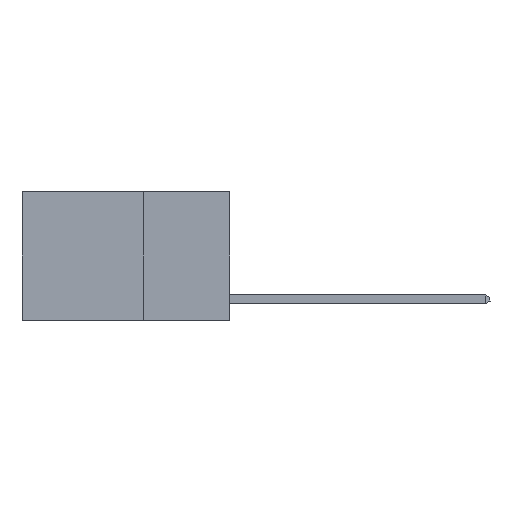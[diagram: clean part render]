
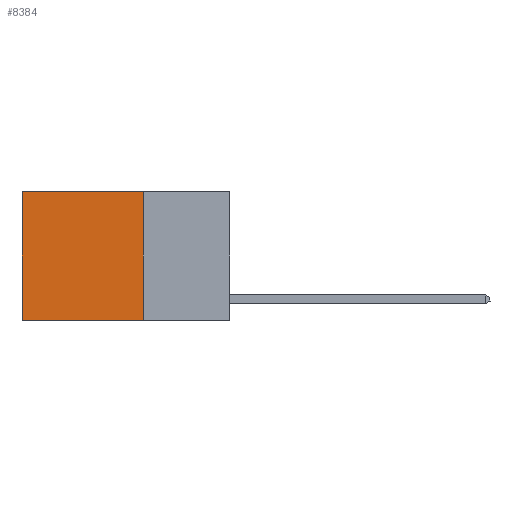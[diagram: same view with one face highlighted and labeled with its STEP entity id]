
A CAD part, left-side view. The second image highlights one B-rep face of the part: STEP entity #8384.
In plain terms, the highlighted planar face has unit normal (-1, 0, 0).
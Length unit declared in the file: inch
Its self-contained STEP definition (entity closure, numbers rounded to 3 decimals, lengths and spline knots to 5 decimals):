
#756 = DIRECTION ( 'NONE',  ( 1., 0., 0. ) ) ;
#1683 = ORIENTED_EDGE ( 'NONE', *, *, #12003, .F. ) ;
#1758 = VECTOR ( 'NONE', #3280, 39.37008 ) ;
#2076 = VECTOR ( 'NONE', #7123, 39.37008 ) ;
#2706 = AXIS2_PLACEMENT_3D ( 'NONE', #3637, #756, #6891 ) ;
#3280 = DIRECTION ( 'NONE',  ( 0., 1., 0. ) ) ;
#3371 = VERTEX_POINT ( 'NONE', #11591 ) ;
#3637 = CARTESIAN_POINT ( 'NONE',  ( 0.2625, 0.25, 0. ) ) ;
#4453 = CARTESIAN_POINT ( 'NONE',  ( 0.2625, 0.6, 0. ) ) ;
#4506 = EDGE_CURVE ( 'NONE', #8704, #18616, #5095, .T. ) ;
#5095 = LINE ( 'NONE', #8259, #14985 ) ;
#5238 = ORIENTED_EDGE ( 'NONE', *, *, #6884, .F. ) ;
#5487 = DIRECTION ( 'NONE',  ( 0., 0., -1. ) ) ;
#6106 = FACE_OUTER_BOUND ( 'NONE', #17831, .T. ) ;
#6315 = PLANE ( 'NONE',  #2706 ) ;
#6414 = ORIENTED_EDGE ( 'NONE', *, *, #12177, .T. ) ;
#6884 = EDGE_CURVE ( 'NONE', #19389, #3371, #13389, .T. ) ;
#6891 = DIRECTION ( 'NONE',  ( 0., 0., -1. ) ) ;
#7123 = DIRECTION ( 'NONE',  ( 0., 1., 0. ) ) ;
#8259 = CARTESIAN_POINT ( 'NONE',  ( 0.2625, 0.6, 0. ) ) ;
#8324 = ORIENTED_EDGE ( 'NONE', *, *, #4506, .T. ) ;
#8384 = ADVANCED_FACE ( 'NONE', ( #6106 ), #6315, .F. ) ;
#8704 = VERTEX_POINT ( 'NONE', #4453 ) ;
#9621 = CARTESIAN_POINT ( 'NONE',  ( 0.2625, 0.25, -0.37 ) ) ;
#10752 = CARTESIAN_POINT ( 'NONE',  ( 0.2625, 0.25, 0. ) ) ;
#11151 = LINE ( 'NONE', #9621, #1758 ) ;
#11591 = CARTESIAN_POINT ( 'NONE',  ( 0.2625, 0.25, -0.37 ) ) ;
#12003 = EDGE_CURVE ( 'NONE', #3371, #18616, #11151, .T. ) ;
#12177 = EDGE_CURVE ( 'NONE', #19389, #8704, #16142, .T. ) ;
#13060 = CARTESIAN_POINT ( 'NONE',  ( 0.2625, 0.25, 0. ) ) ;
#13389 = LINE ( 'NONE', #18424, #18309 ) ;
#14555 = CARTESIAN_POINT ( 'NONE',  ( 0.2625, 0.6, -0.37 ) ) ;
#14985 = VECTOR ( 'NONE', #5487, 39.37008 ) ;
#16142 = LINE ( 'NONE', #13060, #2076 ) ;
#16673 = DIRECTION ( 'NONE',  ( 0., 0., -1. ) ) ;
#17831 = EDGE_LOOP ( 'NONE', ( #8324, #1683, #5238, #6414 ) ) ;
#18309 = VECTOR ( 'NONE', #16673, 39.37008 ) ;
#18424 = CARTESIAN_POINT ( 'NONE',  ( 0.2625, 0.25, 0. ) ) ;
#18616 = VERTEX_POINT ( 'NONE', #14555 ) ;
#19389 = VERTEX_POINT ( 'NONE', #10752 ) ;
